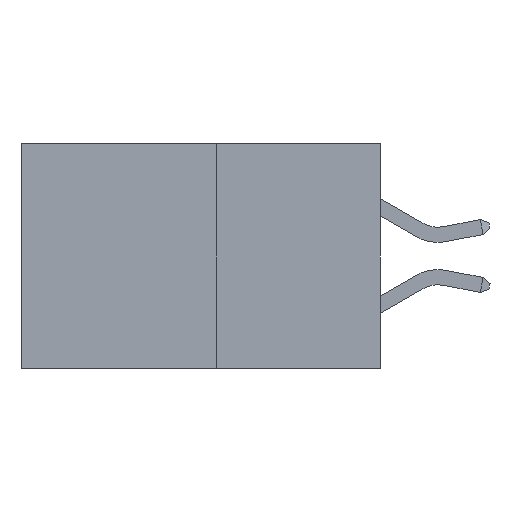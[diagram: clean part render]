
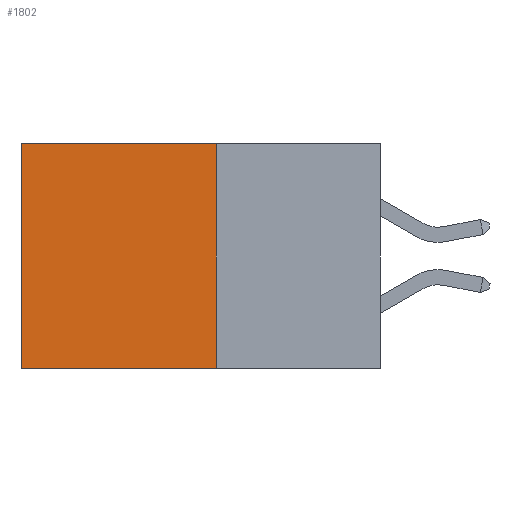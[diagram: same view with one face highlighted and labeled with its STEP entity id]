
A CAD part, left-side view. The second image highlights one B-rep face of the part: STEP entity #1802.
In plain terms, the highlighted planar face has unit normal (-1, 0, 0).
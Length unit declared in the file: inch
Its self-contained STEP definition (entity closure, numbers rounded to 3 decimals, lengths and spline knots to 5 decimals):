
#684 = VERTEX_POINT ( 'NONE', #22922 ) ;
#896 = LINE ( 'NONE', #22834, #4157 ) ;
#929 = CARTESIAN_POINT ( 'NONE',  ( 0.277, 0.27, -0.37 ) ) ;
#1668 = CARTESIAN_POINT ( 'NONE',  ( 0.277, 0.59, -0.37 ) ) ;
#1802 = ADVANCED_FACE ( 'NONE', ( #13998 ), #5449, .F. ) ;
#1833 = ORIENTED_EDGE ( 'NONE', *, *, #3670, .F. ) ;
#2450 = CARTESIAN_POINT ( 'NONE',  ( 0.277, 0.27, -0.37 ) ) ;
#2968 = DIRECTION ( 'NONE',  ( 0., 1., 0. ) ) ;
#3670 = EDGE_CURVE ( 'NONE', #684, #20584, #7337, .T. ) ;
#4157 = VECTOR ( 'NONE', #2968, 39.37008 ) ;
#4725 = VERTEX_POINT ( 'NONE', #20884 ) ;
#5449 = PLANE ( 'NONE',  #16719 ) ;
#7337 = LINE ( 'NONE', #2450, #14732 ) ;
#8554 = ORIENTED_EDGE ( 'NONE', *, *, #13119, .T. ) ;
#9341 = CARTESIAN_POINT ( 'NONE',  ( 0.277, 0.27, -0.37 ) ) ;
#10167 = CARTESIAN_POINT ( 'NONE',  ( 0.277, 0.59, 0. ) ) ;
#10925 = VECTOR ( 'NONE', #16343, 39.37008 ) ;
#11129 = EDGE_LOOP ( 'NONE', ( #16747, #14793, #1833, #8554 ) ) ;
#11783 = VERTEX_POINT ( 'NONE', #10167 ) ;
#12060 = CARTESIAN_POINT ( 'NONE',  ( 0.277, 0.27, -0.37 ) ) ;
#12327 = LINE ( 'NONE', #12060, #17121 ) ;
#13119 = EDGE_CURVE ( 'NONE', #684, #11783, #896, .T. ) ;
#13998 = FACE_OUTER_BOUND ( 'NONE', #11129, .T. ) ;
#14732 = VECTOR ( 'NONE', #16861, 39.37008 ) ;
#14793 = ORIENTED_EDGE ( 'NONE', *, *, #19882, .F. ) ;
#15651 = DIRECTION ( 'NONE',  ( 0., 1., 0. ) ) ;
#15689 = LINE ( 'NONE', #1668, #10925 ) ;
#16343 = DIRECTION ( 'NONE',  ( 0., 0., -1. ) ) ;
#16719 = AXIS2_PLACEMENT_3D ( 'NONE', #9341, #20757, #17979 ) ;
#16747 = ORIENTED_EDGE ( 'NONE', *, *, #22887, .T. ) ;
#16861 = DIRECTION ( 'NONE',  ( 0., 0., -1. ) ) ;
#17121 = VECTOR ( 'NONE', #15651, 39.37008 ) ;
#17979 = DIRECTION ( 'NONE',  ( 0., 0., -1. ) ) ;
#19882 = EDGE_CURVE ( 'NONE', #20584, #4725, #12327, .T. ) ;
#20584 = VERTEX_POINT ( 'NONE', #929 ) ;
#20757 = DIRECTION ( 'NONE',  ( 1., 0., 0. ) ) ;
#20884 = CARTESIAN_POINT ( 'NONE',  ( 0.277, 0.59, -0.37 ) ) ;
#22834 = CARTESIAN_POINT ( 'NONE',  ( 0.277, 0.27, 0. ) ) ;
#22887 = EDGE_CURVE ( 'NONE', #11783, #4725, #15689, .T. ) ;
#22922 = CARTESIAN_POINT ( 'NONE',  ( 0.277, 0.27, 0. ) ) ;
